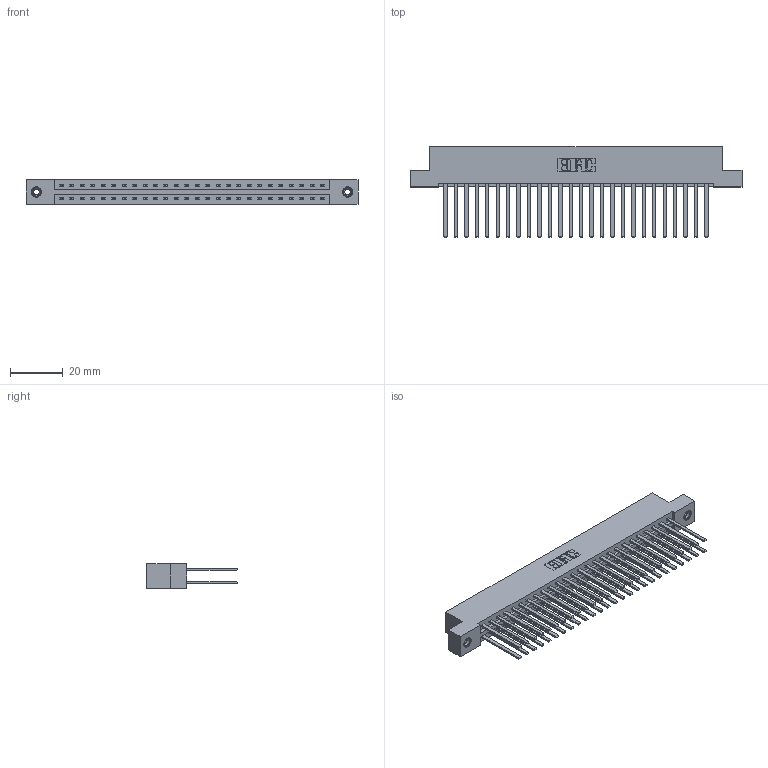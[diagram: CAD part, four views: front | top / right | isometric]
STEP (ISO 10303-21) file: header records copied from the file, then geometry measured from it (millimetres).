
FILE_DESCRIPTION (( 'STEP AP203' ), '1' );
FILE_NAME ('337-052-544-208.STEP', '2018-08-09T23:07:41', ( '' ), ( '' ), 'SwSTEP 2.0', 'SolidWorks 2016', '' );
FILE_SCHEMA (( 'CONFIG_CONTROL_DESIGN' ));
Length unit declared in the file: inch
Products named in the file (4): 337 Part_Flush Mounting Lugs - 0.156 Dia-TI; 345-292-001_345-293-144; 345-250-001_345-250-003-102; 337-052-544-208
Assembly tree (55 placements, depth 2):
  337-052-544-208
    337 Part_Flush Mounting Lugs - 0.156 Dia-TI
    345-292-001_345-293-144  x52
    345-250-001_345-250-003-102  x2
Bounding box: 126.03 x 34.3 x 9.4 mm (x, y, z)
Volume: 13792 mm3; surface area: 17841.7 mm2
Topology: 55 solids, 55 shells, 2670 faces, 7883 edges, 5178 vertices
Faces by surface type: plane 1870, cylinder 784, cone 12, torus 4
Entity records: 23230 total; most frequent: CARTESIAN_POINT 3905, ORIENTED_EDGE 3834, DIRECTION 3379, EDGE_CURVE 1917, VECTOR 1773, LINE 1773, VERTEX_POINT 1272, AXIS2_PLACEMENT_3D 803
